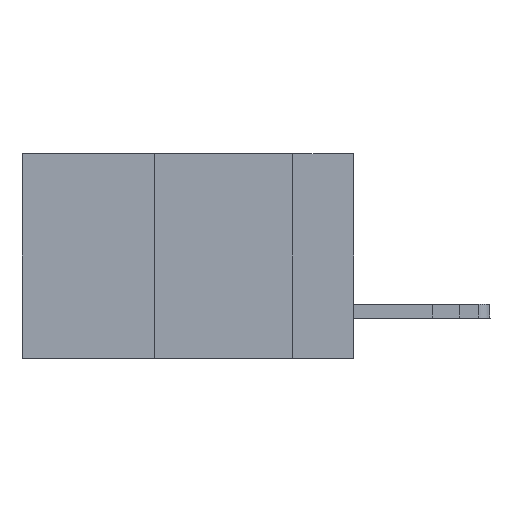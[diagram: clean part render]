
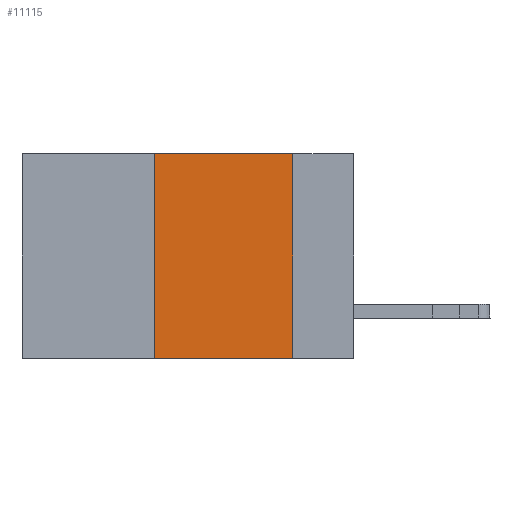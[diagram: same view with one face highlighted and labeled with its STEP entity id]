
A CAD part, left-side view. The second image highlights one B-rep face of the part: STEP entity #11115.
In plain terms, the highlighted planar face has unit normal (-1, 0, 0).
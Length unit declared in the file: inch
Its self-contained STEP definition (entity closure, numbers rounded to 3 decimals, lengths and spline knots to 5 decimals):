
#1180 = VERTEX_POINT ( 'NONE', #13274 ) ;
#1654 = CARTESIAN_POINT ( 'NONE',  ( 0., 0.36, -0.37 ) ) ;
#1862 = DIRECTION ( 'NONE',  ( 0., -1., 0. ) ) ;
#1903 = EDGE_LOOP ( 'NONE', ( #13134, #4753, #10848, #14569 ) ) ;
#2708 = AXIS2_PLACEMENT_3D ( 'NONE', #20240, #12402, #3061 ) ;
#3061 = DIRECTION ( 'NONE',  ( 0., 0., -1. ) ) ;
#4364 = VERTEX_POINT ( 'NONE', #15360 ) ;
#4753 = ORIENTED_EDGE ( 'NONE', *, *, #6094, .F. ) ;
#6094 = EDGE_CURVE ( 'NONE', #8739, #4364, #13149, .T. ) ;
#6257 = DIRECTION ( 'NONE',  ( 0., -1., 0. ) ) ;
#7187 = DIRECTION ( 'NONE',  ( 0., 0., 1. ) ) ;
#7775 = LINE ( 'NONE', #17501, #16018 ) ;
#8140 = DIRECTION ( 'NONE',  ( 0., 0., -1. ) ) ;
#8197 = CARTESIAN_POINT ( 'NONE',  ( 0., 0.36, 0. ) ) ;
#8709 = EDGE_CURVE ( 'NONE', #4364, #1180, #7775, .T. ) ;
#8739 = VERTEX_POINT ( 'NONE', #8197 ) ;
#9493 = VECTOR ( 'NONE', #7187, 39.37008 ) ;
#9975 = LINE ( 'NONE', #10197, #9493 ) ;
#10168 = VECTOR ( 'NONE', #6257, 39.37008 ) ;
#10197 = CARTESIAN_POINT ( 'NONE',  ( 0., 0.36, 0. ) ) ;
#10745 = EDGE_CURVE ( 'NONE', #19386, #8739, #9975, .T. ) ;
#10848 = ORIENTED_EDGE ( 'NONE', *, *, #10745, .F. ) ;
#11115 = ADVANCED_FACE ( 'NONE', ( #16068 ), #18711, .F. ) ;
#11765 = EDGE_CURVE ( 'NONE', #19386, #1180, #14295, .T. ) ;
#12402 = DIRECTION ( 'NONE',  ( 1., 0., 0. ) ) ;
#13134 = ORIENTED_EDGE ( 'NONE', *, *, #8709, .F. ) ;
#13149 = LINE ( 'NONE', #17660, #20508 ) ;
#13274 = CARTESIAN_POINT ( 'NONE',  ( 0., 0.11, -0.37 ) ) ;
#13945 = CARTESIAN_POINT ( 'NONE',  ( 0., 0.6, -0.37 ) ) ;
#14295 = LINE ( 'NONE', #13945, #10168 ) ;
#14569 = ORIENTED_EDGE ( 'NONE', *, *, #11765, .T. ) ;
#15360 = CARTESIAN_POINT ( 'NONE',  ( 0., 0.11, 0. ) ) ;
#16018 = VECTOR ( 'NONE', #8140, 39.37008 ) ;
#16068 = FACE_OUTER_BOUND ( 'NONE', #1903, .T. ) ;
#17501 = CARTESIAN_POINT ( 'NONE',  ( 0., 0.11, 0. ) ) ;
#17660 = CARTESIAN_POINT ( 'NONE',  ( 0., 0.6, 0. ) ) ;
#18711 = PLANE ( 'NONE',  #2708 ) ;
#19386 = VERTEX_POINT ( 'NONE', #1654 ) ;
#20240 = CARTESIAN_POINT ( 'NONE',  ( 0., 0.6, 0. ) ) ;
#20508 = VECTOR ( 'NONE', #1862, 39.37008 ) ;
